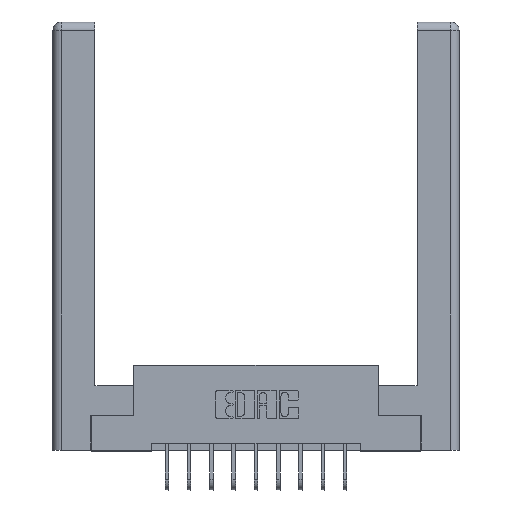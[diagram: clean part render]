
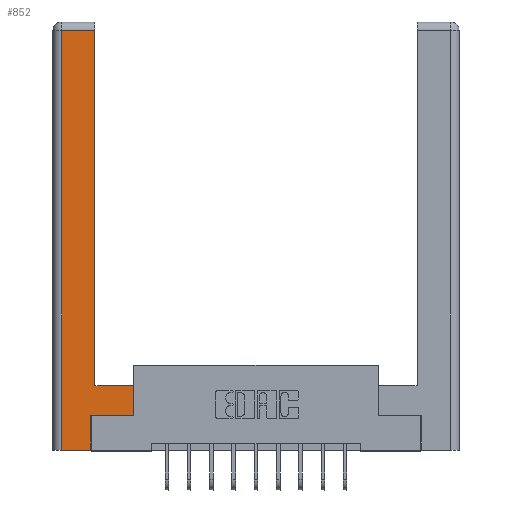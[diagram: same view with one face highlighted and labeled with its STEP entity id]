
A CAD part, top view. The second image highlights one B-rep face of the part: STEP entity #852.
In plain terms, the highlighted planar face has unit normal (0, 0, 1).
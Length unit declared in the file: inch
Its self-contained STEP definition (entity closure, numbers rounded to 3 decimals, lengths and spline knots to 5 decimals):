
#269 = VERTEX_POINT ( 'NONE', #11792 ) ;
#341 = VERTEX_POINT ( 'NONE', #2916 ) ;
#353 = EDGE_CURVE ( 'NONE', #2642, #10585, #5353, .T. ) ;
#811 = PLANE ( 'NONE',  #9579 ) ;
#852 = ADVANCED_FACE ( 'NONE', ( #7643 ), #811, .F. ) ;
#966 = CARTESIAN_POINT ( 'NONE',  ( 0.295, 0.45, 0. ) ) ;
#1570 = CARTESIAN_POINT ( 'NONE',  ( 0.295, 3., 0. ) ) ;
#1763 = LINE ( 'NONE', #4448, #12363 ) ;
#1766 = EDGE_LOOP ( 'NONE', ( #2117, #13569, #11708, #2754, #10333, #7040, #8924, #12578 ) ) ;
#2117 = ORIENTED_EDGE ( 'NONE', *, *, #9281, .T. ) ;
#2238 = LINE ( 'NONE', #9890, #2723 ) ;
#2475 = EDGE_CURVE ( 'NONE', #4504, #9163, #12471, .T. ) ;
#2642 = VERTEX_POINT ( 'NONE', #3568 ) ;
#2723 = VECTOR ( 'NONE', #6657, 39.37008 ) ;
#2724 = CARTESIAN_POINT ( 'NONE',  ( 0.0615, 2.94, 0. ) ) ;
#2754 = ORIENTED_EDGE ( 'NONE', *, *, #8416, .T. ) ;
#2916 = CARTESIAN_POINT ( 'NONE',  ( 0.265, 0., 0. ) ) ;
#3553 = DIRECTION ( 'NONE',  ( 1., 0., 0. ) ) ;
#3568 = CARTESIAN_POINT ( 'NONE',  ( 0.295, 2.94, 0. ) ) ;
#4002 = DIRECTION ( 'NONE',  ( 0., 0., -1. ) ) ;
#4103 = CARTESIAN_POINT ( 'NONE',  ( 0.0615, 0., 0. ) ) ;
#4242 = DIRECTION ( 'NONE',  ( 0., -1., 0. ) ) ;
#4448 = CARTESIAN_POINT ( 'NONE',  ( 0.265, 0., 0. ) ) ;
#4489 = DIRECTION ( 'NONE',  ( 1., 0., 0. ) ) ;
#4504 = VERTEX_POINT ( 'NONE', #6269 ) ;
#5199 = VECTOR ( 'NONE', #3553, 39.37008 ) ;
#5353 = LINE ( 'NONE', #9477, #13470 ) ;
#6269 = CARTESIAN_POINT ( 'NONE',  ( 0.565, 0.245, 0. ) ) ;
#6513 = LINE ( 'NONE', #13100, #5199 ) ;
#6657 = DIRECTION ( 'NONE',  ( -1., 0., 0. ) ) ;
#6763 = DIRECTION ( 'NONE',  ( 0., 1., 0. ) ) ;
#7040 = ORIENTED_EDGE ( 'NONE', *, *, #9036, .T. ) ;
#7227 = VERTEX_POINT ( 'NONE', #966 ) ;
#7643 = FACE_OUTER_BOUND ( 'NONE', #1766, .T. ) ;
#7763 = EDGE_CURVE ( 'NONE', #10585, #12875, #9387, .T. ) ;
#8346 = VECTOR ( 'NONE', #6763, 39.37008 ) ;
#8400 = CARTESIAN_POINT ( 'NONE',  ( 0.0615, 0., 0. ) ) ;
#8416 = EDGE_CURVE ( 'NONE', #12875, #341, #1763, .T. ) ;
#8560 = VECTOR ( 'NONE', #4242, 39.37008 ) ;
#8728 = CARTESIAN_POINT ( 'NONE',  ( 0.565, 0.45, 0. ) ) ;
#8850 = LINE ( 'NONE', #1570, #8346 ) ;
#8924 = ORIENTED_EDGE ( 'NONE', *, *, #2475, .T. ) ;
#9036 = EDGE_CURVE ( 'NONE', #269, #4504, #6513, .T. ) ;
#9163 = VERTEX_POINT ( 'NONE', #8728 ) ;
#9266 = CARTESIAN_POINT ( 'NONE',  ( 0., 0., 0. ) ) ;
#9281 = EDGE_CURVE ( 'NONE', #7227, #2642, #8850, .T. ) ;
#9387 = LINE ( 'NONE', #8400, #8560 ) ;
#9477 = CARTESIAN_POINT ( 'NONE',  ( 0.0615, 2.94, 0. ) ) ;
#9579 = AXIS2_PLACEMENT_3D ( 'NONE', #9266, #4002, #12620 ) ;
#9639 = VECTOR ( 'NONE', #10706, 39.37008 ) ;
#9733 = EDGE_CURVE ( 'NONE', #9163, #7227, #2238, .T. ) ;
#9890 = CARTESIAN_POINT ( 'NONE',  ( 0.295, 0.45, 0. ) ) ;
#10333 = ORIENTED_EDGE ( 'NONE', *, *, #12066, .T. ) ;
#10572 = VECTOR ( 'NONE', #11574, 39.37008 ) ;
#10585 = VERTEX_POINT ( 'NONE', #2724 ) ;
#10706 = DIRECTION ( 'NONE',  ( 0., 1., 0. ) ) ;
#10916 = LINE ( 'NONE', #12316, #10572 ) ;
#11574 = DIRECTION ( 'NONE',  ( 0., 1., 0. ) ) ;
#11708 = ORIENTED_EDGE ( 'NONE', *, *, #7763, .T. ) ;
#11730 = CARTESIAN_POINT ( 'NONE',  ( 0.565, 0.45, 0. ) ) ;
#11792 = CARTESIAN_POINT ( 'NONE',  ( 0.265, 0.245, 0. ) ) ;
#12066 = EDGE_CURVE ( 'NONE', #341, #269, #10916, .T. ) ;
#12316 = CARTESIAN_POINT ( 'NONE',  ( 0.265, 0.245, 0. ) ) ;
#12363 = VECTOR ( 'NONE', #4489, 39.37008 ) ;
#12471 = LINE ( 'NONE', #11730, #9639 ) ;
#12578 = ORIENTED_EDGE ( 'NONE', *, *, #9733, .T. ) ;
#12620 = DIRECTION ( 'NONE',  ( -1., 0., 0. ) ) ;
#12875 = VERTEX_POINT ( 'NONE', #4103 ) ;
#13100 = CARTESIAN_POINT ( 'NONE',  ( 0.565, 0.245, 0. ) ) ;
#13470 = VECTOR ( 'NONE', #13560, 39.37008 ) ;
#13560 = DIRECTION ( 'NONE',  ( -1., 0., 0. ) ) ;
#13569 = ORIENTED_EDGE ( 'NONE', *, *, #353, .T. ) ;
